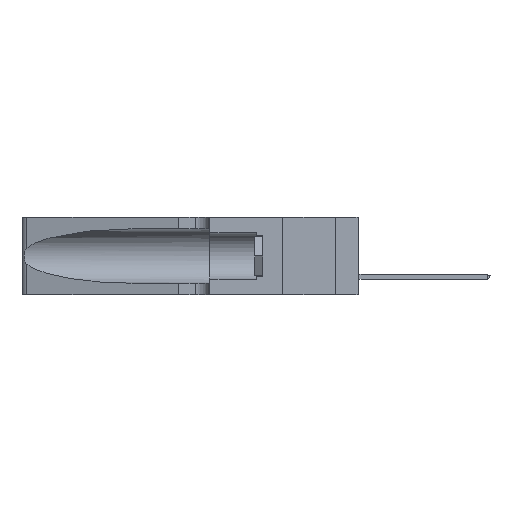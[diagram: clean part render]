
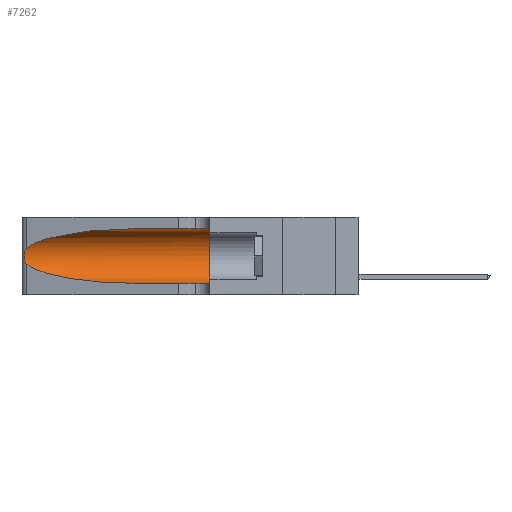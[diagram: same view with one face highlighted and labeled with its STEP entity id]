
A CAD part, left-side view. The second image highlights one B-rep face of the part: STEP entity #7262.
In plain terms, the highlighted cylindrical face has radius 3.308 mm (diameter 6.617 mm), a partial arc.
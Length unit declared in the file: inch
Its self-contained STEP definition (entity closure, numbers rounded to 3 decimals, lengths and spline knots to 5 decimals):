
#300 =( BOUNDED_CURVE ( )  B_SPLINE_CURVE ( 3, ( #34641, #31023, #11071, #7291 ),
 .UNSPECIFIED., .F., .F. ) 
 B_SPLINE_CURVE_WITH_KNOTS ( ( 4, 4 ),
 ( 3.44316, 4.71239 ),
 .UNSPECIFIED. ) 
 CURVE ( )  GEOMETRIC_REPRESENTATION_ITEM ( )  RATIONAL_B_SPLINE_CURVE ( ( 1., 0.87, 0.87, 1. ) ) 
 REPRESENTATION_ITEM ( '' )  );
#1054 = ORIENTED_EDGE ( 'NONE', *, *, #23205, .T. ) ;
#1397 = VERTEX_POINT ( 'NONE', #35095 ) ;
#2075 = DIRECTION ( 'NONE',  ( 0., 1., 0. ) ) ;
#5412 = CARTESIAN_POINT ( 'NONE',  ( 0.1305, 1.61858, 0.05475 ) ) ;
#5939 = CARTESIAN_POINT ( 'NONE',  ( 0.26075, 1.23896, 0.19203 ) ) ;
#7036 = CARTESIAN_POINT ( 'NONE',  ( 0.1305, 1.61858, 0.185 ) ) ;
#7112 = CARTESIAN_POINT ( 'NONE',  ( 0.25487, 1.22718, 0.22369 ) ) ;
#7262 = ADVANCED_FACE ( 'NONE', ( #24243 ), #25435, .F. ) ;
#7291 = CARTESIAN_POINT ( 'NONE',  ( 0.1305, 0.72297, 0.05475 ) ) ;
#8669 = EDGE_LOOP ( 'NONE', ( #23177, #29321, #11590, #1054, #35497, #46164 ) ) ;
#9576 = DIRECTION ( 'NONE',  ( 0., -1., 0. ) ) ;
#10063 = CARTESIAN_POINT ( 'NONE',  ( 0.1305, 0.35, 0.185 ) ) ;
#10517 = CARTESIAN_POINT ( 'NONE',  ( 0.26075, 1.23896, 0.178 ) ) ;
#10699 = CARTESIAN_POINT ( 'NONE',  ( 0.25487, 1.22718, 0.14631 ) ) ;
#11071 = CARTESIAN_POINT ( 'NONE',  ( 0.18966, 0.96281, 0.05475 ) ) ;
#11116 = EDGE_CURVE ( 'NONE', #14544, #23127, #45654, .T. ) ;
#11590 = ORIENTED_EDGE ( 'NONE', *, *, #13990, .T. ) ;
#11777 = VECTOR ( 'NONE', #9576, 39.37008 ) ;
#12583 = VERTEX_POINT ( 'NONE', #41947 ) ;
#13037 = AXIS2_PLACEMENT_3D ( 'NONE', #7036, #31139, #50613 ) ;
#13464 = EDGE_CURVE ( 'NONE', #14544, #21111, #28817, .T. ) ;
#13990 = EDGE_CURVE ( 'NONE', #47899, #1397, #300, .T. ) ;
#14109 = CARTESIAN_POINT ( 'NONE',  ( 0.25639, 1.23184, 0.21858 ) ) ;
#14544 = VERTEX_POINT ( 'NONE', #19020 ) ;
#17344 = CARTESIAN_POINT ( 'NONE',  ( 0.25487, 1.22718, 0.22369 ) ) ;
#17927 = CARTESIAN_POINT ( 'NONE',  ( 0.25856, 1.23593, 0.16098 ) ) ;
#18358 = VECTOR ( 'NONE', #32022, 39.37008 ) ;
#18704 = CARTESIAN_POINT ( 'NONE',  ( 0.25555, 1.22994, 0.2215 ) ) ;
#19020 = CARTESIAN_POINT ( 'NONE',  ( 0.1305, 0.72297, 0.31525 ) ) ;
#21111 = VERTEX_POINT ( 'NONE', #39574 ) ;
#21278 = DIRECTION ( 'NONE',  ( 0., 0., 1. ) ) ;
#21909 = CARTESIAN_POINT ( 'NONE',  ( 0.25789, 1.23486, 0.15765 ) ) ;
#22100 = CARTESIAN_POINT ( 'NONE',  ( 0.26018, 1.23835, 0.19895 ) ) ;
#23127 = VERTEX_POINT ( 'NONE', #7112 ) ;
#23177 = ORIENTED_EDGE ( 'NONE', *, *, #11116, .T. ) ;
#23205 = EDGE_CURVE ( 'NONE', #1397, #12583, #50099, .T. ) ;
#24243 = FACE_OUTER_BOUND ( 'NONE', #8669, .T. ) ;
#24431 = AXIS2_PLACEMENT_3D ( 'NONE', #10063, #2075, #21278 ) ;
#25435 = CYLINDRICAL_SURFACE ( 'NONE', #13037, 0.13025 ) ;
#27684 = CARTESIAN_POINT ( 'NONE',  ( 0.25487, 1.22718, 0.14631 ) ) ;
#28817 = LINE ( 'NONE', #32719, #18358 ) ;
#29162 = CARTESIAN_POINT ( 'NONE',  ( 0.1305, 0.72297, 0.31525 ) ) ;
#29321 = ORIENTED_EDGE ( 'NONE', *, *, #33638, .T. ) ;
#30292 = CARTESIAN_POINT ( 'NONE',  ( 0.25639, 1.23186, 0.15144 ) ) ;
#31023 = CARTESIAN_POINT ( 'NONE',  ( 0.2373, 1.15595, 0.08982 ) ) ;
#31139 = DIRECTION ( 'NONE',  ( 0., -1., 0. ) ) ;
#32022 = DIRECTION ( 'NONE',  ( 0., -1., 0. ) ) ;
#32719 = CARTESIAN_POINT ( 'NONE',  ( 0.1305, 1.61858, 0.31525 ) ) ;
#33292 = B_SPLINE_CURVE_WITH_KNOTS ( 'NONE', 3,
 ( #42023, #18704, #14109, #46129, #41635, #22100, #5939, #10517, #38241, #17927, #21909, #30292, #45577, #10699 ),
 .UNSPECIFIED., .F., .F.,
 ( 4, 2, 2, 2, 2, 2, 4 ),
 ( 0., 0.00027, 0.00053, 0.00107, 0.0016, 0.00187, 0.00214 ),
 .UNSPECIFIED. ) ;
#33638 = EDGE_CURVE ( 'NONE', #23127, #47899, #33292, .T. ) ;
#34641 = CARTESIAN_POINT ( 'NONE',  ( 0.25487, 1.22718, 0.14631 ) ) ;
#35095 = CARTESIAN_POINT ( 'NONE',  ( 0.1305, 0.72297, 0.05475 ) ) ;
#35497 = ORIENTED_EDGE ( 'NONE', *, *, #45715, .F. ) ;
#38241 = CARTESIAN_POINT ( 'NONE',  ( 0.26017, 1.23833, 0.17102 ) ) ;
#39574 = CARTESIAN_POINT ( 'NONE',  ( 0.1305, 0.35, 0.31525 ) ) ;
#41080 = CARTESIAN_POINT ( 'NONE',  ( 0.2373, 1.15595, 0.28018 ) ) ;
#41635 = CARTESIAN_POINT ( 'NONE',  ( 0.25854, 1.2359, 0.20912 ) ) ;
#41769 = CIRCLE ( 'NONE', #24431, 0.13025 ) ;
#41947 = CARTESIAN_POINT ( 'NONE',  ( 0.1305, 0.35, 0.05475 ) ) ;
#42023 = CARTESIAN_POINT ( 'NONE',  ( 0.25487, 1.22718, 0.22369 ) ) ;
#45577 = CARTESIAN_POINT ( 'NONE',  ( 0.25555, 1.22993, 0.14849 ) ) ;
#45654 =( BOUNDED_CURVE ( )  B_SPLINE_CURVE ( 3, ( #29162, #48578, #41080, #17344 ),
 .UNSPECIFIED., .F., .F. ) 
 B_SPLINE_CURVE_WITH_KNOTS ( ( 4, 4 ),
 ( 1.5708, 2.84003 ),
 .UNSPECIFIED. ) 
 CURVE ( )  GEOMETRIC_REPRESENTATION_ITEM ( )  RATIONAL_B_SPLINE_CURVE ( ( 1., 0.87, 0.87, 1. ) ) 
 REPRESENTATION_ITEM ( '' )  );
#45715 = EDGE_CURVE ( 'NONE', #21111, #12583, #41769, .T. ) ;
#46129 = CARTESIAN_POINT ( 'NONE',  ( 0.25787, 1.23484, 0.2124 ) ) ;
#46164 = ORIENTED_EDGE ( 'NONE', *, *, #13464, .F. ) ;
#47899 = VERTEX_POINT ( 'NONE', #27684 ) ;
#48578 = CARTESIAN_POINT ( 'NONE',  ( 0.18966, 0.96281, 0.31525 ) ) ;
#50099 = LINE ( 'NONE', #5412, #11777 ) ;
#50613 = DIRECTION ( 'NONE',  ( 0., 0., -1. ) ) ;
